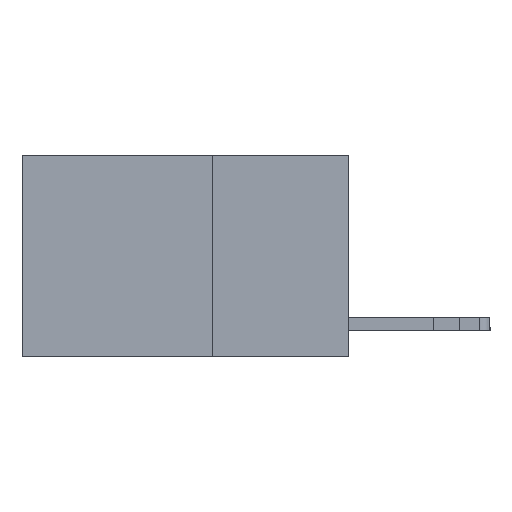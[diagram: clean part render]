
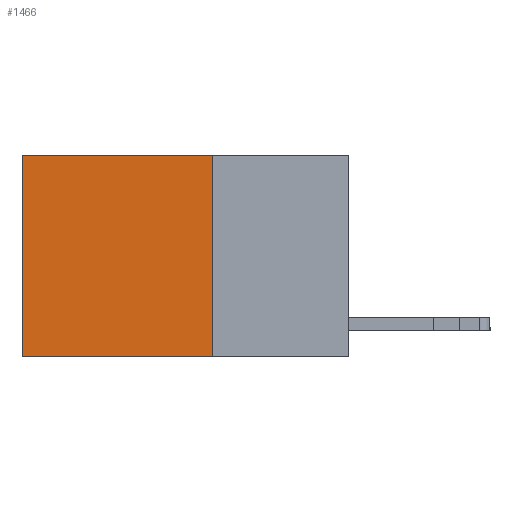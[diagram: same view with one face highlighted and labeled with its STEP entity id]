
A CAD part, left-side view. The second image highlights one B-rep face of the part: STEP entity #1466.
In plain terms, the highlighted planar face has unit normal (-1, 0, 0).
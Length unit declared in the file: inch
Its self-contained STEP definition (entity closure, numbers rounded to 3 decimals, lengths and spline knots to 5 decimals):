
#342 = EDGE_CURVE ( 'NONE', #6413, #6263, #6738, .T. ) ;
#1051 = VECTOR ( 'NONE', #5823, 39.37008 ) ;
#1466 = ADVANCED_FACE ( 'NONE', ( #12291 ), #3093, .F. ) ;
#1790 = DIRECTION ( 'NONE',  ( 0., 0., -1. ) ) ;
#1861 = ORIENTED_EDGE ( 'NONE', *, *, #8650, .F. ) ;
#1873 = CARTESIAN_POINT ( 'NONE',  ( 0.2625, 0.6, 0. ) ) ;
#1967 = VERTEX_POINT ( 'NONE', #2298 ) ;
#1971 = ORIENTED_EDGE ( 'NONE', *, *, #4733, .F. ) ;
#2100 = CARTESIAN_POINT ( 'NONE',  ( 0.2625, 0.6, -0.37 ) ) ;
#2298 = CARTESIAN_POINT ( 'NONE',  ( 0.2625, 0.25, -0.37 ) ) ;
#3093 = PLANE ( 'NONE',  #5453 ) ;
#3225 = LINE ( 'NONE', #9922, #9443 ) ;
#3501 = EDGE_LOOP ( 'NONE', ( #3756, #1861, #1971, #4098 ) ) ;
#3756 = ORIENTED_EDGE ( 'NONE', *, *, #342, .T. ) ;
#4075 = CARTESIAN_POINT ( 'NONE',  ( 0.2625, 0.25, 0. ) ) ;
#4098 = ORIENTED_EDGE ( 'NONE', *, *, #4417, .T. ) ;
#4122 = DIRECTION ( 'NONE',  ( 1., 0., 0. ) ) ;
#4417 = EDGE_CURVE ( 'NONE', #6631, #6413, #3225, .T. ) ;
#4697 = LINE ( 'NONE', #12621, #11974 ) ;
#4733 = EDGE_CURVE ( 'NONE', #6631, #1967, #4697, .T. ) ;
#5453 = AXIS2_PLACEMENT_3D ( 'NONE', #6251, #4122, #7242 ) ;
#5823 = DIRECTION ( 'NONE',  ( 0., 0., -1. ) ) ;
#6001 = DIRECTION ( 'NONE',  ( 0., 1., 0. ) ) ;
#6251 = CARTESIAN_POINT ( 'NONE',  ( 0.2625, 0.25, 0. ) ) ;
#6263 = VERTEX_POINT ( 'NONE', #2100 ) ;
#6413 = VERTEX_POINT ( 'NONE', #12341 ) ;
#6631 = VERTEX_POINT ( 'NONE', #4075 ) ;
#6738 = LINE ( 'NONE', #1873, #1051 ) ;
#7242 = DIRECTION ( 'NONE',  ( 0., 0., -1. ) ) ;
#7564 = DIRECTION ( 'NONE',  ( 0., 1., 0. ) ) ;
#8650 = EDGE_CURVE ( 'NONE', #1967, #6263, #9780, .T. ) ;
#8727 = VECTOR ( 'NONE', #7564, 39.37008 ) ;
#9443 = VECTOR ( 'NONE', #6001, 39.37008 ) ;
#9780 = LINE ( 'NONE', #10514, #8727 ) ;
#9922 = CARTESIAN_POINT ( 'NONE',  ( 0.2625, 0.25, 0. ) ) ;
#10514 = CARTESIAN_POINT ( 'NONE',  ( 0.2625, 0.25, -0.37 ) ) ;
#11974 = VECTOR ( 'NONE', #1790, 39.37008 ) ;
#12291 = FACE_OUTER_BOUND ( 'NONE', #3501, .T. ) ;
#12341 = CARTESIAN_POINT ( 'NONE',  ( 0.2625, 0.6, 0. ) ) ;
#12621 = CARTESIAN_POINT ( 'NONE',  ( 0.2625, 0.25, 0. ) ) ;
